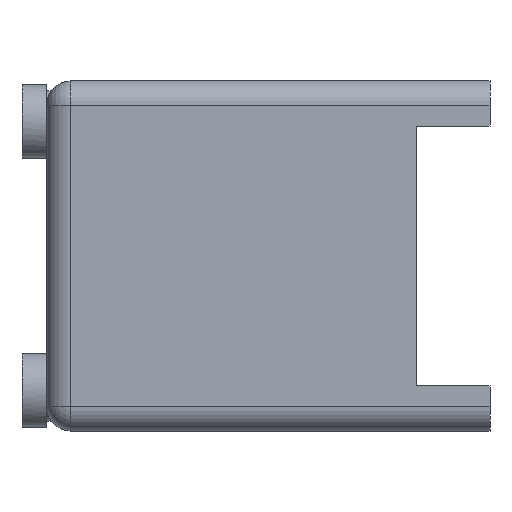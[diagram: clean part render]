
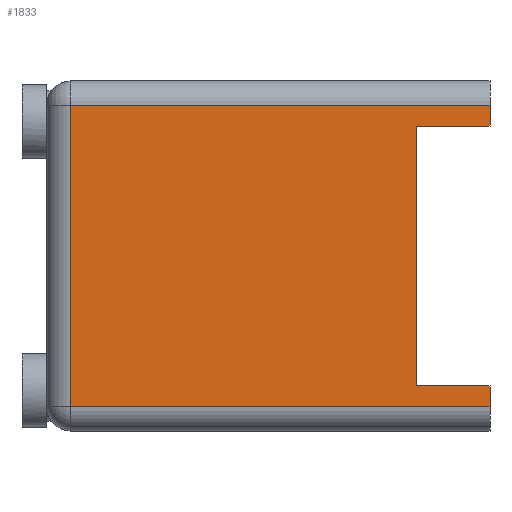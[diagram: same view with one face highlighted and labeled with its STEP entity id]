
A CAD part, left-side view. The second image highlights one B-rep face of the part: STEP entity #1833.
In plain terms, the highlighted planar face has unit normal (-1, 0, 0).
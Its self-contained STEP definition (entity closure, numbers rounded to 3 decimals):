
#22 = VERTEX_POINT ( 'NONE', #701 ) ;
#33 = CARTESIAN_POINT ( 'NONE',  ( 0., 3.81, -2.337 ) ) ;
#60 = DIRECTION ( 'NONE',  ( 0., 0., 1. ) ) ;
#64 = AXIS2_PLACEMENT_3D ( 'NONE', #1379, #1553, #111 ) ;
#66 = EDGE_CURVE ( 'NONE', #22, #516, #397, .T. ) ;
#84 = CARTESIAN_POINT ( 'NONE',  ( 0., 0., -18.161 ) ) ;
#110 = ORIENTED_EDGE ( 'NONE', *, *, #238, .F. ) ;
#111 = DIRECTION ( 'NONE',  ( 0., 0., 1. ) ) ;
#175 = ORIENTED_EDGE ( 'NONE', *, *, #772, .T. ) ;
#181 = ORIENTED_EDGE ( 'NONE', *, *, #66, .T. ) ;
#184 = DIRECTION ( 'NONE',  ( 0., -1., 0. ) ) ;
#238 = EDGE_CURVE ( 'NONE', #1177, #983, #1527, .T. ) ;
#289 = VERTEX_POINT ( 'NONE', #1689 ) ;
#320 = ORIENTED_EDGE ( 'NONE', *, *, #980, .T. ) ;
#397 = LINE ( 'NONE', #942, #928 ) ;
#468 = ORIENTED_EDGE ( 'NONE', *, *, #1384, .F. ) ;
#516 = VERTEX_POINT ( 'NONE', #2080 ) ;
#584 = LINE ( 'NONE', #33, #862 ) ;
#587 = VECTOR ( 'NONE', #184, 1000. ) ;
#681 = EDGE_CURVE ( 'NONE', #22, #1177, #584, .T. ) ;
#701 = CARTESIAN_POINT ( 'NONE',  ( 0., 0., -2.337 ) ) ;
#723 = VECTOR ( 'NONE', #2037, 1000. ) ;
#772 = EDGE_CURVE ( 'NONE', #516, #1245, #1577, .T. ) ;
#790 = CARTESIAN_POINT ( 'NONE',  ( 0., 3.81, -15.824 ) ) ;
#817 = VECTOR ( 'NONE', #1670, 1000. ) ;
#819 = EDGE_CURVE ( 'NONE', #1245, #2077, #1214, .T. ) ;
#849 = CARTESIAN_POINT ( 'NONE',  ( 0., 23.012, -1.27 ) ) ;
#862 = VECTOR ( 'NONE', #2160, 1000. ) ;
#870 = CARTESIAN_POINT ( 'NONE',  ( 0., 0., -15.824 ) ) ;
#872 = CARTESIAN_POINT ( 'NONE',  ( 0., 21.742, -18.161 ) ) ;
#928 = VECTOR ( 'NONE', #60, 1000. ) ;
#942 = CARTESIAN_POINT ( 'NONE',  ( 0., 0., -18.161 ) ) ;
#962 = LINE ( 'NONE', #2183, #817 ) ;
#980 = EDGE_CURVE ( 'NONE', #2077, #289, #962, .T. ) ;
#983 = VERTEX_POINT ( 'NONE', #790 ) ;
#1013 = LINE ( 'NONE', #84, #1884 ) ;
#1167 = EDGE_CURVE ( 'NONE', #289, #1882, #1013, .T. ) ;
#1177 = VERTEX_POINT ( 'NONE', #1538 ) ;
#1185 = CARTESIAN_POINT ( 'NONE',  ( 0., 3.81, -15.824 ) ) ;
#1204 = CARTESIAN_POINT ( 'NONE',  ( 0., 3.81, -15.824 ) ) ;
#1214 = LINE ( 'NONE', #872, #1321 ) ;
#1245 = VERTEX_POINT ( 'NONE', #1329 ) ;
#1321 = VECTOR ( 'NONE', #1363, 1000. ) ;
#1329 = CARTESIAN_POINT ( 'NONE',  ( 0., 21.742, -1.27 ) ) ;
#1363 = DIRECTION ( 'NONE',  ( 0., 0., -1. ) ) ;
#1379 = CARTESIAN_POINT ( 'NONE',  ( 0., 0., -18.161 ) ) ;
#1384 = EDGE_CURVE ( 'NONE', #983, #1882, #1936, .T. ) ;
#1390 = PLANE ( 'NONE',  #64 ) ;
#1396 = ORIENTED_EDGE ( 'NONE', *, *, #1167, .T. ) ;
#1421 = ORIENTED_EDGE ( 'NONE', *, *, #681, .F. ) ;
#1488 = CARTESIAN_POINT ( 'NONE',  ( 0., 21.742, -16.891 ) ) ;
#1527 = LINE ( 'NONE', #1185, #723 ) ;
#1538 = CARTESIAN_POINT ( 'NONE',  ( 0., 3.81, -2.337 ) ) ;
#1553 = DIRECTION ( 'NONE',  ( -1., 0., 0. ) ) ;
#1577 = LINE ( 'NONE', #849, #1611 ) ;
#1611 = VECTOR ( 'NONE', #2247, 1000. ) ;
#1670 = DIRECTION ( 'NONE',  ( 0., -1., 0. ) ) ;
#1689 = CARTESIAN_POINT ( 'NONE',  ( 0., 0., -16.891 ) ) ;
#1700 = FACE_OUTER_BOUND ( 'NONE', #1879, .T. ) ;
#1746 = ORIENTED_EDGE ( 'NONE', *, *, #819, .T. ) ;
#1833 = ADVANCED_FACE ( 'NONE', ( #1700 ), #1390, .T. ) ;
#1879 = EDGE_LOOP ( 'NONE', ( #1746, #320, #1396, #468, #110, #1421, #181, #175 ) ) ;
#1882 = VERTEX_POINT ( 'NONE', #870 ) ;
#1884 = VECTOR ( 'NONE', #2210, 1000. ) ;
#1936 = LINE ( 'NONE', #1204, #587 ) ;
#2037 = DIRECTION ( 'NONE',  ( 0., 0., -1. ) ) ;
#2077 = VERTEX_POINT ( 'NONE', #1488 ) ;
#2080 = CARTESIAN_POINT ( 'NONE',  ( 0., 0., -1.27 ) ) ;
#2160 = DIRECTION ( 'NONE',  ( 0., 1., 0. ) ) ;
#2183 = CARTESIAN_POINT ( 'NONE',  ( 0., 0., -16.891 ) ) ;
#2210 = DIRECTION ( 'NONE',  ( 0., 0., 1. ) ) ;
#2247 = DIRECTION ( 'NONE',  ( 0., 1., 0. ) ) ;
